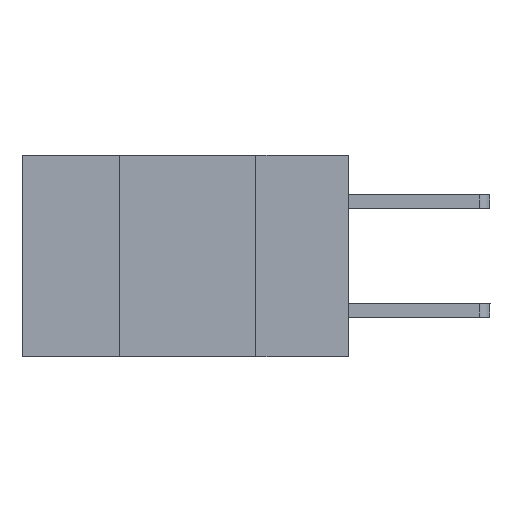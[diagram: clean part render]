
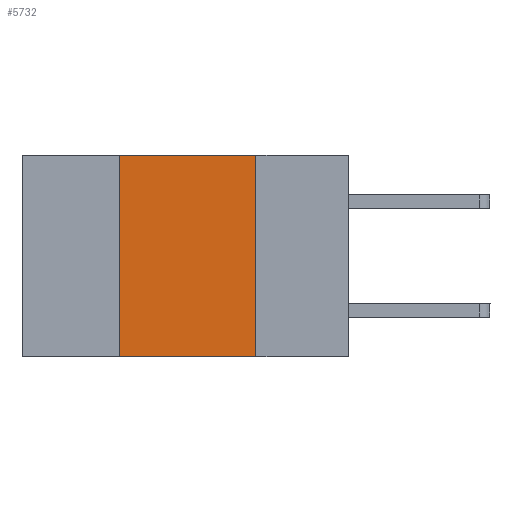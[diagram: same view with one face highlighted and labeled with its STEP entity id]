
A CAD part, left-side view. The second image highlights one B-rep face of the part: STEP entity #5732.
In plain terms, the highlighted planar face has unit normal (-1, 0, 0).
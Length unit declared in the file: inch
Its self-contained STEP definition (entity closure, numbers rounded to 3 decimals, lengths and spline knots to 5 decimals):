
#121 = DIRECTION ( 'NONE',  ( 0., 0., -1. ) ) ;
#123 = ORIENTED_EDGE ( 'NONE', *, *, #3984, .F. ) ;
#137 = CARTESIAN_POINT ( 'NONE',  ( 0., 0.42, -0.37 ) ) ;
#260 = CARTESIAN_POINT ( 'NONE',  ( 0., 0.17, -0.37 ) ) ;
#287 = LINE ( 'NONE', #137, #2302 ) ;
#412 = VERTEX_POINT ( 'NONE', #4174 ) ;
#1285 = EDGE_CURVE ( 'NONE', #4531, #3290, #8707, .T. ) ;
#1434 = ORIENTED_EDGE ( 'NONE', *, *, #2198, .F. ) ;
#2130 = LINE ( 'NONE', #2356, #5864 ) ;
#2183 = VERTEX_POINT ( 'NONE', #5322 ) ;
#2198 = EDGE_CURVE ( 'NONE', #4531, #412, #287, .T. ) ;
#2302 = VECTOR ( 'NONE', #8681, 39.37008 ) ;
#2341 = DIRECTION ( 'NONE',  ( 0., -1., 0. ) ) ;
#2356 = CARTESIAN_POINT ( 'NONE',  ( 0., 0.6, 0. ) ) ;
#2741 = VECTOR ( 'NONE', #121, 39.37008 ) ;
#3290 = VERTEX_POINT ( 'NONE', #5428 ) ;
#3610 = DIRECTION ( 'NONE',  ( 1., 0., 0. ) ) ;
#3787 = FACE_OUTER_BOUND ( 'NONE', #5917, .T. ) ;
#3984 = EDGE_CURVE ( 'NONE', #2183, #3290, #7172, .T. ) ;
#4174 = CARTESIAN_POINT ( 'NONE',  ( 0., 0.42, 0. ) ) ;
#4531 = VERTEX_POINT ( 'NONE', #9242 ) ;
#5322 = CARTESIAN_POINT ( 'NONE',  ( 0., 0.17, 0. ) ) ;
#5428 = CARTESIAN_POINT ( 'NONE',  ( 0., 0.17, -0.37 ) ) ;
#5434 = EDGE_CURVE ( 'NONE', #412, #2183, #2130, .T. ) ;
#5732 = ADVANCED_FACE ( 'NONE', ( #3787 ), #6563, .F. ) ;
#5864 = VECTOR ( 'NONE', #2341, 39.37008 ) ;
#5917 = EDGE_LOOP ( 'NONE', ( #123, #6856, #1434, #7137 ) ) ;
#6535 = VECTOR ( 'NONE', #9270, 39.37008 ) ;
#6563 = PLANE ( 'NONE',  #8311 ) ;
#6856 = ORIENTED_EDGE ( 'NONE', *, *, #5434, .F. ) ;
#7137 = ORIENTED_EDGE ( 'NONE', *, *, #1285, .T. ) ;
#7172 = LINE ( 'NONE', #260, #2741 ) ;
#8045 = CARTESIAN_POINT ( 'NONE',  ( 0., 0.6, 0. ) ) ;
#8311 = AXIS2_PLACEMENT_3D ( 'NONE', #8045, #3610, #8768 ) ;
#8681 = DIRECTION ( 'NONE',  ( 0., 0., 1. ) ) ;
#8707 = LINE ( 'NONE', #8928, #6535 ) ;
#8768 = DIRECTION ( 'NONE',  ( 0., 0., -1. ) ) ;
#8928 = CARTESIAN_POINT ( 'NONE',  ( 0., 0.6, -0.37 ) ) ;
#9242 = CARTESIAN_POINT ( 'NONE',  ( 0., 0.42, -0.37 ) ) ;
#9270 = DIRECTION ( 'NONE',  ( 0., -1., 0. ) ) ;
